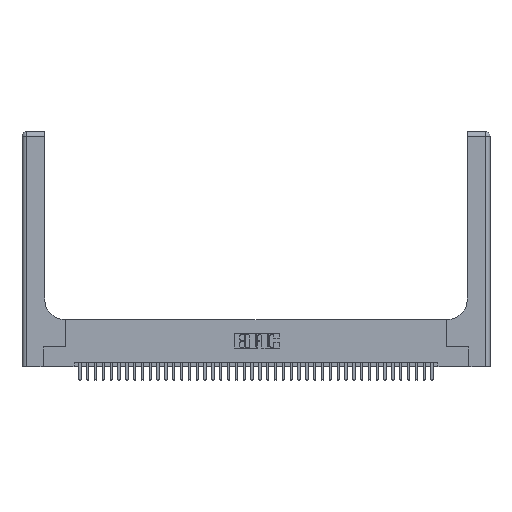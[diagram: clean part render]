
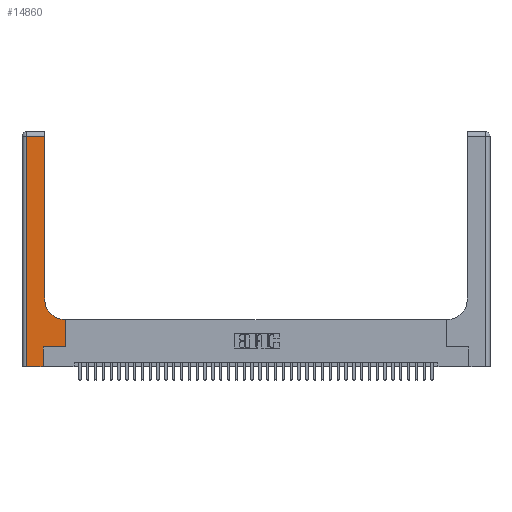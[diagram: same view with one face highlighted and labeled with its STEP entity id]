
A CAD part, top view. The second image highlights one B-rep face of the part: STEP entity #14860.
In plain terms, the highlighted planar face has unit normal (0, 0, 1).
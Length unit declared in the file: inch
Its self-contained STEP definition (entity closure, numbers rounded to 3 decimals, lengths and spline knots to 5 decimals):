
#848 = DIRECTION ( 'NONE',  ( -1., 0., 0. ) ) ;
#1697 = ORIENTED_EDGE ( 'NONE', *, *, #16357, .T. ) ;
#2097 = AXIS2_PLACEMENT_3D ( 'NONE', #29077, #13328, #32359 ) ;
#2214 = EDGE_CURVE ( 'NONE', #30420, #20516, #34043, .T. ) ;
#2327 = ORIENTED_EDGE ( 'NONE', *, *, #31351, .T. ) ;
#3820 = LINE ( 'NONE', #38614, #36482 ) ;
#3822 = VERTEX_POINT ( 'NONE', #18575 ) ;
#6536 = VERTEX_POINT ( 'NONE', #35879 ) ;
#7018 = DIRECTION ( 'NONE',  ( 0., -1., 0. ) ) ;
#7419 = VECTOR ( 'NONE', #33663, 39.37008 ) ;
#7735 = LINE ( 'NONE', #14379, #40351 ) ;
#7923 = CARTESIAN_POINT ( 'NONE',  ( 0.5585, 0.6, 0.37 ) ) ;
#10322 = FACE_OUTER_BOUND ( 'NONE', #15160, .T. ) ;
#10546 = VERTEX_POINT ( 'NONE', #24220 ) ;
#10564 = VECTOR ( 'NONE', #34101, 39.37008 ) ;
#10599 = DIRECTION ( 'NONE',  ( 0., 0., -1. ) ) ;
#11148 = VECTOR ( 'NONE', #27568, 39.37008 ) ;
#12259 = EDGE_CURVE ( 'NONE', #20516, #28404, #13529, .T. ) ;
#12902 = CARTESIAN_POINT ( 'NONE',  ( 0.2915, 0.6, 0.37 ) ) ;
#13328 = DIRECTION ( 'NONE',  ( 0., 0., -1. ) ) ;
#13529 = LINE ( 'NONE', #15049, #10564 ) ;
#13895 = ORIENTED_EDGE ( 'NONE', *, *, #19230, .T. ) ;
#14068 = LINE ( 'NONE', #12902, #40222 ) ;
#14379 = CARTESIAN_POINT ( 'NONE',  ( 0.269, 0., 0.37 ) ) ;
#14858 = LINE ( 'NONE', #23754, #40022 ) ;
#14860 = ADVANCED_FACE ( 'NONE', ( #10322 ), #38287, .F. ) ;
#15049 = CARTESIAN_POINT ( 'NONE',  ( 0.5585, 0.25, 0.37 ) ) ;
#15134 = CARTESIAN_POINT ( 'NONE',  ( 0.269, 0.25, 0.37 ) ) ;
#15160 = EDGE_LOOP ( 'NONE', ( #21063, #13895, #23927, #40215, #28408, #25827, #21802, #2327, #1697 ) ) ;
#15620 = CARTESIAN_POINT ( 'NONE',  ( 0.269, 0.25, 0.37 ) ) ;
#15944 = EDGE_CURVE ( 'NONE', #36107, #39500, #3820, .T. ) ;
#16357 = EDGE_CURVE ( 'NONE', #6536, #30341, #31508, .T. ) ;
#16497 = DIRECTION ( 'NONE',  ( 1., 0., 0. ) ) ;
#17014 = LINE ( 'NONE', #36948, #11148 ) ;
#17427 = CARTESIAN_POINT ( 'NONE',  ( 0.06, 0., 0.37 ) ) ;
#17833 = EDGE_CURVE ( 'NONE', #30341, #3822, #17014, .T. ) ;
#18575 = CARTESIAN_POINT ( 'NONE',  ( 0.2915, 2.94, 0.37 ) ) ;
#19230 = EDGE_CURVE ( 'NONE', #3822, #36107, #14858, .T. ) ;
#20512 = CARTESIAN_POINT ( 'NONE',  ( 0.2915, 0.85, 0.37 ) ) ;
#20516 = VERTEX_POINT ( 'NONE', #20824 ) ;
#20705 = DIRECTION ( 'NONE',  ( -1., 0., 0. ) ) ;
#20824 = CARTESIAN_POINT ( 'NONE',  ( 0.5585, 0.25, 0.37 ) ) ;
#21063 = ORIENTED_EDGE ( 'NONE', *, *, #17833, .T. ) ;
#21802 = ORIENTED_EDGE ( 'NONE', *, *, #12259, .T. ) ;
#22347 = EDGE_CURVE ( 'NONE', #10546, #30420, #7735, .T. ) ;
#23754 = CARTESIAN_POINT ( 'NONE',  ( 0., 2.94, 0.37 ) ) ;
#23927 = ORIENTED_EDGE ( 'NONE', *, *, #15944, .T. ) ;
#24220 = CARTESIAN_POINT ( 'NONE',  ( 0.269, 0., 0.37 ) ) ;
#25251 = CARTESIAN_POINT ( 'NONE',  ( 0.5415, 0.85, 0.37 ) ) ;
#25827 = ORIENTED_EDGE ( 'NONE', *, *, #2214, .T. ) ;
#27238 = LINE ( 'NONE', #27737, #7419 ) ;
#27568 = DIRECTION ( 'NONE',  ( 0., 1., 0. ) ) ;
#27737 = CARTESIAN_POINT ( 'NONE',  ( 0., 0., 0.37 ) ) ;
#27772 = EDGE_CURVE ( 'NONE', #39500, #10546, #27238, .T. ) ;
#28136 = DIRECTION ( 'NONE',  ( 1., 0., 0. ) ) ;
#28404 = VERTEX_POINT ( 'NONE', #7923 ) ;
#28408 = ORIENTED_EDGE ( 'NONE', *, *, #22347, .T. ) ;
#28865 = AXIS2_PLACEMENT_3D ( 'NONE', #25251, #10599, #16497 ) ;
#29077 = CARTESIAN_POINT ( 'NONE',  ( 0., 3., 0.37 ) ) ;
#29346 = CARTESIAN_POINT ( 'NONE',  ( 0.06, 2.94, 0.37 ) ) ;
#29803 = DIRECTION ( 'NONE',  ( 0., 1., 0. ) ) ;
#30341 = VERTEX_POINT ( 'NONE', #20512 ) ;
#30420 = VERTEX_POINT ( 'NONE', #15620 ) ;
#31351 = EDGE_CURVE ( 'NONE', #28404, #6536, #14068, .T. ) ;
#31508 = CIRCLE ( 'NONE', #28865, 0.25 ) ;
#31568 = VECTOR ( 'NONE', #28136, 39.37008 ) ;
#32359 = DIRECTION ( 'NONE',  ( -1., 0., 0. ) ) ;
#33663 = DIRECTION ( 'NONE',  ( 1., 0., 0. ) ) ;
#34043 = LINE ( 'NONE', #15134, #31568 ) ;
#34101 = DIRECTION ( 'NONE',  ( 0., 1., 0. ) ) ;
#35879 = CARTESIAN_POINT ( 'NONE',  ( 0.5415, 0.6, 0.37 ) ) ;
#36107 = VERTEX_POINT ( 'NONE', #29346 ) ;
#36482 = VECTOR ( 'NONE', #7018, 39.37008 ) ;
#36948 = CARTESIAN_POINT ( 'NONE',  ( 0.2915, 3., 0.37 ) ) ;
#38287 = PLANE ( 'NONE',  #2097 ) ;
#38614 = CARTESIAN_POINT ( 'NONE',  ( 0.06, 3., 0.37 ) ) ;
#39500 = VERTEX_POINT ( 'NONE', #17427 ) ;
#40022 = VECTOR ( 'NONE', #20705, 39.37008 ) ;
#40215 = ORIENTED_EDGE ( 'NONE', *, *, #27772, .T. ) ;
#40222 = VECTOR ( 'NONE', #848, 39.37008 ) ;
#40351 = VECTOR ( 'NONE', #29803, 39.37008 ) ;
